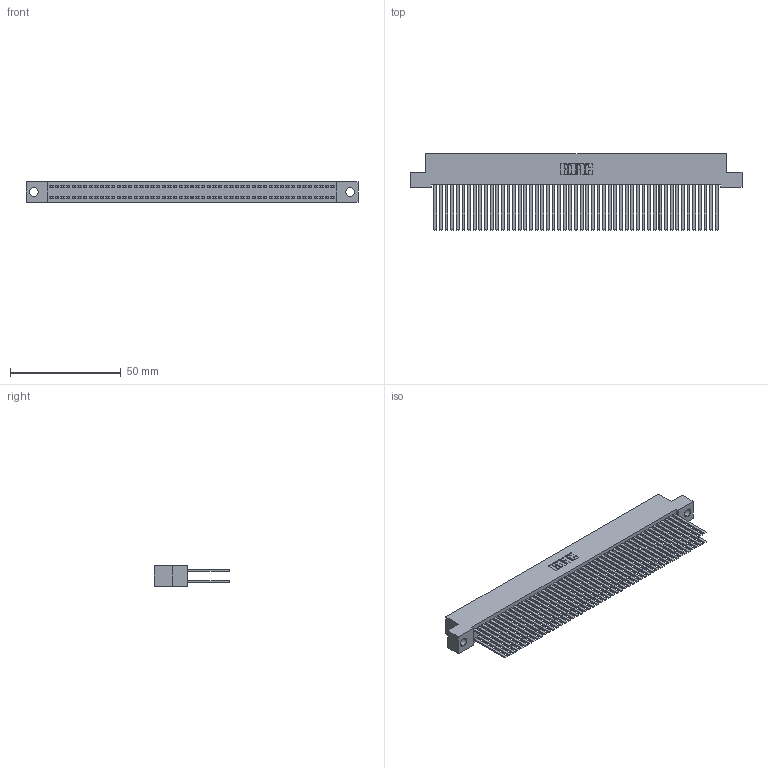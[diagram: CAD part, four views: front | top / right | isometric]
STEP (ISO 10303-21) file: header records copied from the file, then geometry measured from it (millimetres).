
FILE_DESCRIPTION (( 'STEP AP203' ), '1' );
FILE_NAME ('392-102-544-204.STEP', '2019-10-09T21:31:06', ( '' ), ( '' ), 'SwSTEP 2.0', 'SolidWorks 2016', '' );
FILE_SCHEMA (( 'CONFIG_CONTROL_DESIGN' ));
Length unit declared in the file: inch
Products named in the file (3): 342 Part_.156 TH; 345-292-001_345-293-144; 392-102-544-204
Assembly tree (103 placements, depth 2):
  392-102-544-204
    342 Part_.156 TH
    345-292-001_345-293-144  x102
Bounding box: 149.86 x 34.3 x 9.4 mm (x, y, z)
Volume: 14850.3 mm3; surface area: 28178.3 mm2
Topology: 103 solids, 103 shells, 4802 faces, 14273 edges, 9378 vertices
Faces by surface type: plane 3330, cylinder 1472
Entity records: 31333 total; most frequent: CARTESIAN_POINT 5178, ORIENTED_EDGE 5114, DIRECTION 4405, EDGE_CURVE 2557, VECTOR 2433, LINE 2433, VERTEX_POINT 1702, AXIS2_PLACEMENT_3D 986
